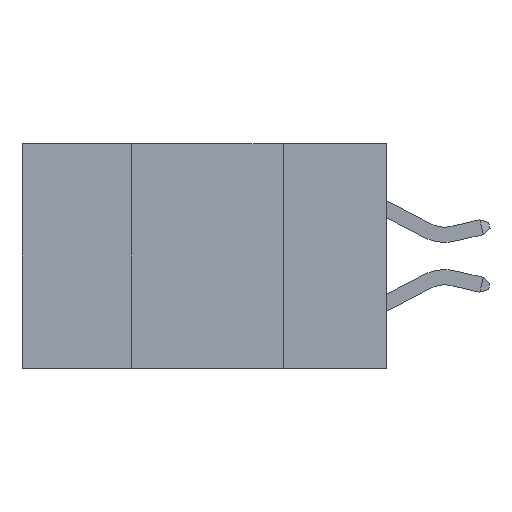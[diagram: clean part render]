
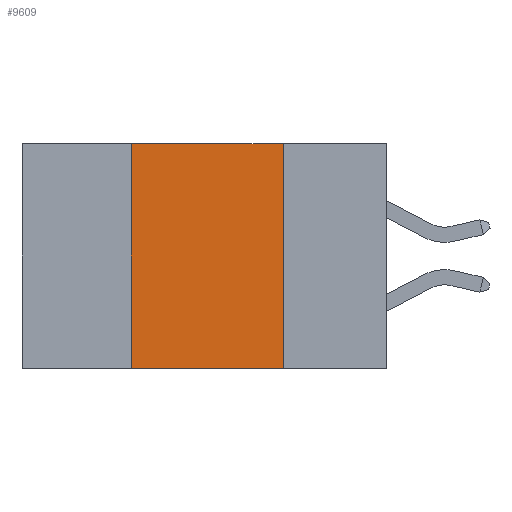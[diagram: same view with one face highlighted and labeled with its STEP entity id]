
A CAD part, left-side view. The second image highlights one B-rep face of the part: STEP entity #9609.
In plain terms, the highlighted planar face has unit normal (-1, 0, 0).
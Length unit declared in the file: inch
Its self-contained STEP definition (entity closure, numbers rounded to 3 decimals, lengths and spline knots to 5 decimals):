
#450 = LINE ( 'NONE', #4432, #7199 ) ;
#593 = EDGE_CURVE ( 'NONE', #15012, #7954, #4705, .T. ) ;
#987 = EDGE_CURVE ( 'NONE', #5047, #11033, #7628, .T. ) ;
#1135 = DIRECTION ( 'NONE',  ( 0., 0., -1. ) ) ;
#1459 = VECTOR ( 'NONE', #14719, 39.37008 ) ;
#1766 = CARTESIAN_POINT ( 'NONE',  ( 0., 0.42, -0.37 ) ) ;
#1767 = LINE ( 'NONE', #6029, #9227 ) ;
#1924 = AXIS2_PLACEMENT_3D ( 'NONE', #15351, #9376, #1135 ) ;
#3238 = ORIENTED_EDGE ( 'NONE', *, *, #9658, .T. ) ;
#3385 = ORIENTED_EDGE ( 'NONE', *, *, #593, .F. ) ;
#3451 = CARTESIAN_POINT ( 'NONE',  ( 0., 0.17, -0.37 ) ) ;
#4000 = CARTESIAN_POINT ( 'NONE',  ( 0., 0.17, 0. ) ) ;
#4432 = CARTESIAN_POINT ( 'NONE',  ( 0., 0.6, 0. ) ) ;
#4705 = LINE ( 'NONE', #8783, #10229 ) ;
#5047 = VERTEX_POINT ( 'NONE', #8287 ) ;
#5381 = DIRECTION ( 'NONE',  ( 0., 0., 1. ) ) ;
#5789 = DIRECTION ( 'NONE',  ( 0., -1., 0. ) ) ;
#5946 = PLANE ( 'NONE',  #1924 ) ;
#6029 = CARTESIAN_POINT ( 'NONE',  ( 0., 0.6, -0.37 ) ) ;
#7199 = VECTOR ( 'NONE', #9339, 39.37008 ) ;
#7628 = LINE ( 'NONE', #4000, #1459 ) ;
#7954 = VERTEX_POINT ( 'NONE', #11400 ) ;
#8287 = CARTESIAN_POINT ( 'NONE',  ( 0., 0.17, 0. ) ) ;
#8396 = ORIENTED_EDGE ( 'NONE', *, *, #987, .F. ) ;
#8783 = CARTESIAN_POINT ( 'NONE',  ( 0., 0.42, 0. ) ) ;
#9227 = VECTOR ( 'NONE', #5789, 39.37008 ) ;
#9339 = DIRECTION ( 'NONE',  ( 0., -1., 0. ) ) ;
#9361 = EDGE_CURVE ( 'NONE', #7954, #5047, #450, .T. ) ;
#9376 = DIRECTION ( 'NONE',  ( 1., 0., 0. ) ) ;
#9606 = FACE_OUTER_BOUND ( 'NONE', #11553, .T. ) ;
#9609 = ADVANCED_FACE ( 'NONE', ( #9606 ), #5946, .F. ) ;
#9658 = EDGE_CURVE ( 'NONE', #15012, #11033, #1767, .T. ) ;
#10229 = VECTOR ( 'NONE', #5381, 39.37008 ) ;
#11033 = VERTEX_POINT ( 'NONE', #3451 ) ;
#11400 = CARTESIAN_POINT ( 'NONE',  ( 0., 0.42, 0. ) ) ;
#11553 = EDGE_LOOP ( 'NONE', ( #8396, #12991, #3385, #3238 ) ) ;
#12991 = ORIENTED_EDGE ( 'NONE', *, *, #9361, .F. ) ;
#14719 = DIRECTION ( 'NONE',  ( 0., 0., -1. ) ) ;
#15012 = VERTEX_POINT ( 'NONE', #1766 ) ;
#15351 = CARTESIAN_POINT ( 'NONE',  ( 0., 0.6, 0. ) ) ;
